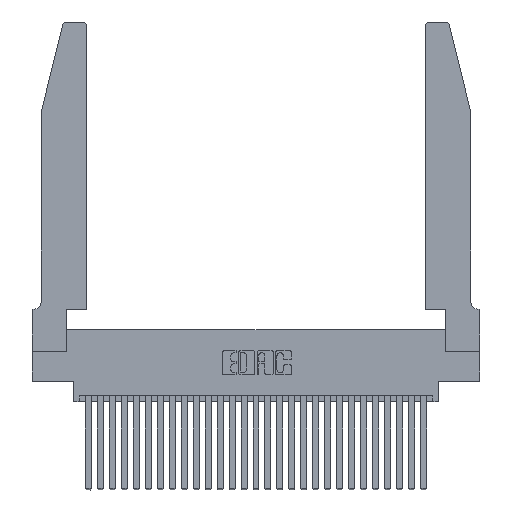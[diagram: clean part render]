
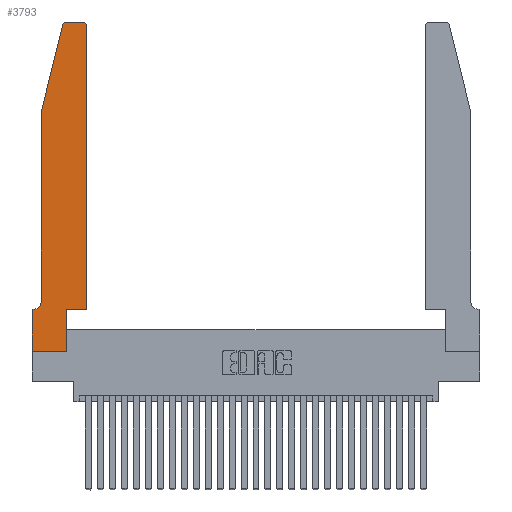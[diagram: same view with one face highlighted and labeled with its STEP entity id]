
A CAD part, top view. The second image highlights one B-rep face of the part: STEP entity #3793.
In plain terms, the highlighted planar face has unit normal (0, 0, 1).
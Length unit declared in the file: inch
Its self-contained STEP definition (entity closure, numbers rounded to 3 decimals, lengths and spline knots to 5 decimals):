
#326 = EDGE_CURVE ( 'NONE', #11363, #2331, #24061, .T. ) ;
#906 = VECTOR ( 'NONE', #25761, 39.37008 ) ;
#926 = CARTESIAN_POINT ( 'NONE',  ( 0.284, 2.72, 0.37 ) ) ;
#1200 = VECTOR ( 'NONE', #13892, 39.37008 ) ;
#1280 = DIRECTION ( 'NONE',  ( 1., 0., 0. ) ) ;
#1293 = CARTESIAN_POINT ( 'NONE',  ( 0.0755, 2., 0.37 ) ) ;
#1429 = PLANE ( 'NONE',  #25523 ) ;
#1620 = VECTOR ( 'NONE', #19970, 39.37008 ) ;
#1793 = CARTESIAN_POINT ( 'NONE',  ( 0.2605, 2.75, 0.37 ) ) ;
#2331 = VERTEX_POINT ( 'NONE', #11325 ) ;
#3086 = EDGE_CURVE ( 'NONE', #25192, #16083, #19012, .T. ) ;
#3501 = EDGE_CURVE ( 'NONE', #19077, #11363, #20770, .T. ) ;
#3735 = DIRECTION ( 'NONE',  ( -1., 0., 0. ) ) ;
#3793 = ADVANCED_FACE ( 'NONE', ( #16854 ), #1429, .T. ) ;
#4303 = CARTESIAN_POINT ( 'NONE',  ( 0.0055, 0.42, 0.37 ) ) ;
#5446 = CARTESIAN_POINT ( 'NONE',  ( 0.0755, 0.35, 0.37 ) ) ;
#5746 = DIRECTION ( 'NONE',  ( -0.239, -0.971, 0. ) ) ;
#5879 = EDGE_CURVE ( 'NONE', #18391, #14402, #22405, .T. ) ;
#6019 = DIRECTION ( 'NONE',  ( 0., 0., 1. ) ) ;
#6033 = VECTOR ( 'NONE', #5746, 39.37008 ) ;
#6074 = LINE ( 'NONE', #19197, #8928 ) ;
#6549 = CARTESIAN_POINT ( 'NONE',  ( 0.4505, 0.35, 0.37 ) ) ;
#6632 = LINE ( 'NONE', #9142, #26777 ) ;
#6814 = DIRECTION ( 'NONE',  ( -1., 0., 0. ) ) ;
#7108 = CARTESIAN_POINT ( 'NONE',  ( 0.0755, 2., 0.37 ) ) ;
#7778 = VECTOR ( 'NONE', #18552, 39.37008 ) ;
#7836 = ORIENTED_EDGE ( 'NONE', *, *, #13668, .T. ) ;
#8928 = VECTOR ( 'NONE', #24130, 39.37008 ) ;
#9049 = DIRECTION ( 'NONE',  ( 0., -1., 0. ) ) ;
#9142 = CARTESIAN_POINT ( 'NONE',  ( 0., 0., 0.37 ) ) ;
#9320 = CARTESIAN_POINT ( 'NONE',  ( 0., 0., 0.37 ) ) ;
#9705 = EDGE_LOOP ( 'NONE', ( #18274, #23489, #7836, #25378, #22728, #13927, #29023, #11834, #22000, #29137, #21328, #13370 ) ) ;
#10080 = CARTESIAN_POINT ( 'NONE',  ( 0.4205, 2.72, 0.37 ) ) ;
#10119 = VERTEX_POINT ( 'NONE', #18680 ) ;
#10293 = CARTESIAN_POINT ( 'NONE',  ( 0.4505, 0.35, 0.37 ) ) ;
#11325 = CARTESIAN_POINT ( 'NONE',  ( 0.284, 2.75, 0.37 ) ) ;
#11363 = VERTEX_POINT ( 'NONE', #20556 ) ;
#11805 = CARTESIAN_POINT ( 'NONE',  ( 0.2865, 0., 0.37 ) ) ;
#11834 = ORIENTED_EDGE ( 'NONE', *, *, #23182, .T. ) ;
#12051 = VECTOR ( 'NONE', #3735, 39.37008 ) ;
#12400 = DIRECTION ( 'NONE',  ( 1., 0., 0. ) ) ;
#12410 = CARTESIAN_POINT ( 'NONE',  ( 0.0755, 2., 0.37 ) ) ;
#12738 = LINE ( 'NONE', #1293, #6033 ) ;
#12770 = AXIS2_PLACEMENT_3D ( 'NONE', #926, #28208, #12400 ) ;
#13258 = CARTESIAN_POINT ( 'NONE',  ( 0.0055, 0.35, 0.37 ) ) ;
#13370 = ORIENTED_EDGE ( 'NONE', *, *, #3501, .T. ) ;
#13668 = EDGE_CURVE ( 'NONE', #10119, #28499, #12738, .T. ) ;
#13892 = DIRECTION ( 'NONE',  ( 1., 0., 0. ) ) ;
#13927 = ORIENTED_EDGE ( 'NONE', *, *, #5879, .T. ) ;
#13982 = CARTESIAN_POINT ( 'NONE',  ( 0.4505, 2.72, 0.37 ) ) ;
#14402 = VERTEX_POINT ( 'NONE', #21111 ) ;
#15711 = DIRECTION ( 'NONE',  ( 0., 0., 1. ) ) ;
#16083 = VERTEX_POINT ( 'NONE', #6549 ) ;
#16498 = CARTESIAN_POINT ( 'NONE',  ( 0.2865, 0.35, 0.37 ) ) ;
#16549 = VERTEX_POINT ( 'NONE', #22855 ) ;
#16854 = FACE_OUTER_BOUND ( 'NONE', #9705, .T. ) ;
#18025 = AXIS2_PLACEMENT_3D ( 'NONE', #4303, #29076, #6814 ) ;
#18136 = AXIS2_PLACEMENT_3D ( 'NONE', #10080, #6019, #23582 ) ;
#18274 = ORIENTED_EDGE ( 'NONE', *, *, #326, .T. ) ;
#18391 = VERTEX_POINT ( 'NONE', #13258 ) ;
#18498 = LINE ( 'NONE', #28993, #1620 ) ;
#18552 = DIRECTION ( 'NONE',  ( 0., -1., 0. ) ) ;
#18645 = VERTEX_POINT ( 'NONE', #11805 ) ;
#18680 = CARTESIAN_POINT ( 'NONE',  ( 0.25487, 2.72718, 0.37 ) ) ;
#19012 = LINE ( 'NONE', #10293, #20447 ) ;
#19077 = VERTEX_POINT ( 'NONE', #13982 ) ;
#19197 = CARTESIAN_POINT ( 'NONE',  ( 0.2865, 0.35, 0.37 ) ) ;
#19228 = EDGE_CURVE ( 'NONE', #28499, #28523, #24051, .T. ) ;
#19970 = DIRECTION ( 'NONE',  ( 0., 1., 0. ) ) ;
#20447 = VECTOR ( 'NONE', #1280, 39.37008 ) ;
#20556 = CARTESIAN_POINT ( 'NONE',  ( 0.4205, 2.75, 0.37 ) ) ;
#20770 = CIRCLE ( 'NONE', #18136, 0.03 ) ;
#21111 = CARTESIAN_POINT ( 'NONE',  ( 0., 0.35, 0.37 ) ) ;
#21198 = CARTESIAN_POINT ( 'NONE',  ( 0.0755, 0.42, 0.37 ) ) ;
#21328 = ORIENTED_EDGE ( 'NONE', *, *, #21987, .T. ) ;
#21987 = EDGE_CURVE ( 'NONE', #16083, #19077, #18498, .T. ) ;
#22000 = ORIENTED_EDGE ( 'NONE', *, *, #22778, .T. ) ;
#22405 = LINE ( 'NONE', #5446, #906 ) ;
#22728 = ORIENTED_EDGE ( 'NONE', *, *, #23689, .T. ) ;
#22778 = EDGE_CURVE ( 'NONE', #18645, #25192, #6074, .T. ) ;
#22855 = CARTESIAN_POINT ( 'NONE',  ( 0., 0., 0.37 ) ) ;
#23182 = EDGE_CURVE ( 'NONE', #16549, #18645, #23715, .T. ) ;
#23489 = ORIENTED_EDGE ( 'NONE', *, *, #27864, .T. ) ;
#23582 = DIRECTION ( 'NONE',  ( 1., 0., 0. ) ) ;
#23689 = EDGE_CURVE ( 'NONE', #28523, #18391, #27237, .T. ) ;
#23715 = LINE ( 'NONE', #9320, #1200 ) ;
#24051 = LINE ( 'NONE', #7108, #7778 ) ;
#24061 = LINE ( 'NONE', #1793, #12051 ) ;
#24130 = DIRECTION ( 'NONE',  ( 0., 1., 0. ) ) ;
#24979 = DIRECTION ( 'NONE',  ( 1., 0., 0. ) ) ;
#25192 = VERTEX_POINT ( 'NONE', #16498 ) ;
#25378 = ORIENTED_EDGE ( 'NONE', *, *, #19228, .T. ) ;
#25523 = AXIS2_PLACEMENT_3D ( 'NONE', #29202, #15711, #24979 ) ;
#25761 = DIRECTION ( 'NONE',  ( -1., 0., 0. ) ) ;
#26777 = VECTOR ( 'NONE', #9049, 39.37008 ) ;
#27237 = CIRCLE ( 'NONE', #18025, 0.07 ) ;
#27864 = EDGE_CURVE ( 'NONE', #2331, #10119, #28591, .T. ) ;
#28208 = DIRECTION ( 'NONE',  ( 0., 0., 1. ) ) ;
#28323 = EDGE_CURVE ( 'NONE', #14402, #16549, #6632, .T. ) ;
#28499 = VERTEX_POINT ( 'NONE', #12410 ) ;
#28523 = VERTEX_POINT ( 'NONE', #21198 ) ;
#28591 = CIRCLE ( 'NONE', #12770, 0.03 ) ;
#28993 = CARTESIAN_POINT ( 'NONE',  ( 0.4505, 0.35, 0.37 ) ) ;
#29023 = ORIENTED_EDGE ( 'NONE', *, *, #28323, .T. ) ;
#29076 = DIRECTION ( 'NONE',  ( 0., 0., -1. ) ) ;
#29137 = ORIENTED_EDGE ( 'NONE', *, *, #3086, .T. ) ;
#29202 = CARTESIAN_POINT ( 'NONE',  ( 0., 0.35, 0.37 ) ) ;
